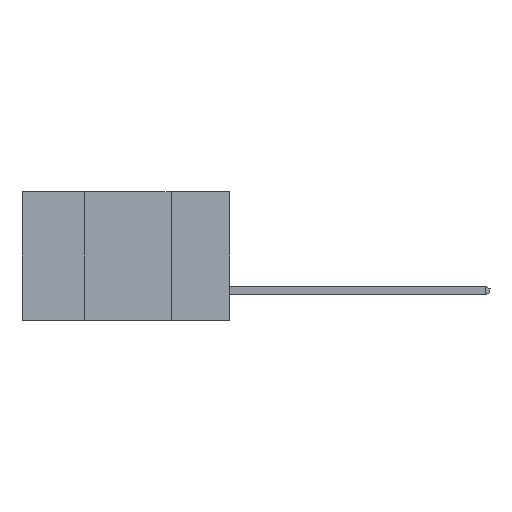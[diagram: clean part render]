
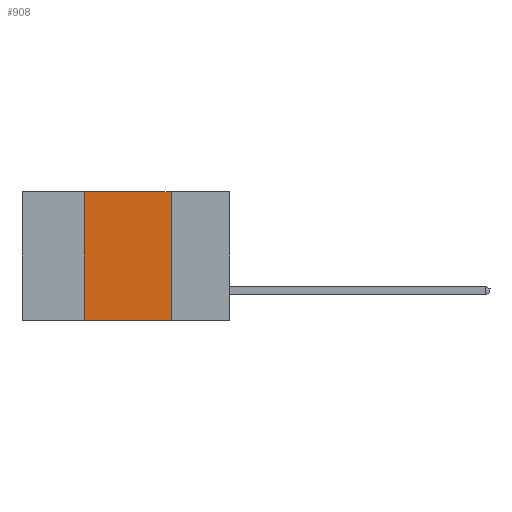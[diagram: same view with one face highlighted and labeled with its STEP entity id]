
A CAD part, left-side view. The second image highlights one B-rep face of the part: STEP entity #908.
In plain terms, the highlighted planar face has unit normal (-1, 0, 0).
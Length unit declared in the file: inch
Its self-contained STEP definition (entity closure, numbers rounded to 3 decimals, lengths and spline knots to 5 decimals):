
#31 = VECTOR ( 'NONE', #11476, 39.37008 ) ;
#45 = CARTESIAN_POINT ( 'NONE',  ( 0., 0.6, 0. ) ) ;
#130 = DIRECTION ( 'NONE',  ( 0., -1., 0. ) ) ;
#282 = DIRECTION ( 'NONE',  ( 1., 0., 0. ) ) ;
#642 = ORIENTED_EDGE ( 'NONE', *, *, #8441, .F. ) ;
#729 = VERTEX_POINT ( 'NONE', #10998 ) ;
#908 = ADVANCED_FACE ( 'NONE', ( #8521 ), #3707, .F. ) ;
#1066 = AXIS2_PLACEMENT_3D ( 'NONE', #45, #282, #9264 ) ;
#1299 = LINE ( 'NONE', #3276, #2844 ) ;
#1772 = VECTOR ( 'NONE', #130, 39.37008 ) ;
#1928 = VECTOR ( 'NONE', #2684, 39.37008 ) ;
#2484 = CARTESIAN_POINT ( 'NONE',  ( 0., 0.42, 0. ) ) ;
#2684 = DIRECTION ( 'NONE',  ( 0., 0., 1. ) ) ;
#2844 = VECTOR ( 'NONE', #10394, 39.37008 ) ;
#2966 = CARTESIAN_POINT ( 'NONE',  ( 0., 0.42, -0.37 ) ) ;
#3188 = EDGE_CURVE ( 'NONE', #4169, #10572, #4189, .T. ) ;
#3276 = CARTESIAN_POINT ( 'NONE',  ( 0., 0.17, -0.37 ) ) ;
#3707 = PLANE ( 'NONE',  #1066 ) ;
#4169 = VERTEX_POINT ( 'NONE', #2966 ) ;
#4189 = LINE ( 'NONE', #8060, #31 ) ;
#4389 = LINE ( 'NONE', #8175, #1928 ) ;
#4517 = EDGE_CURVE ( 'NONE', #5537, #729, #4759, .T. ) ;
#4759 = LINE ( 'NONE', #10196, #1772 ) ;
#5537 = VERTEX_POINT ( 'NONE', #2484 ) ;
#6926 = ORIENTED_EDGE ( 'NONE', *, *, #3188, .T. ) ;
#8060 = CARTESIAN_POINT ( 'NONE',  ( 0., 0.6, -0.37 ) ) ;
#8170 = EDGE_CURVE ( 'NONE', #4169, #5537, #4389, .T. ) ;
#8175 = CARTESIAN_POINT ( 'NONE',  ( 0., 0.42, -0.37 ) ) ;
#8215 = ORIENTED_EDGE ( 'NONE', *, *, #4517, .F. ) ;
#8441 = EDGE_CURVE ( 'NONE', #729, #10572, #1299, .T. ) ;
#8521 = FACE_OUTER_BOUND ( 'NONE', #9529, .T. ) ;
#9264 = DIRECTION ( 'NONE',  ( 0., 0., -1. ) ) ;
#9529 = EDGE_LOOP ( 'NONE', ( #642, #8215, #10529, #6926 ) ) ;
#10196 = CARTESIAN_POINT ( 'NONE',  ( 0., 0.6, 0. ) ) ;
#10394 = DIRECTION ( 'NONE',  ( 0., 0., -1. ) ) ;
#10529 = ORIENTED_EDGE ( 'NONE', *, *, #8170, .F. ) ;
#10572 = VERTEX_POINT ( 'NONE', #11249 ) ;
#10998 = CARTESIAN_POINT ( 'NONE',  ( 0., 0.17, 0. ) ) ;
#11249 = CARTESIAN_POINT ( 'NONE',  ( 0., 0.17, -0.37 ) ) ;
#11476 = DIRECTION ( 'NONE',  ( 0., -1., 0. ) ) ;
